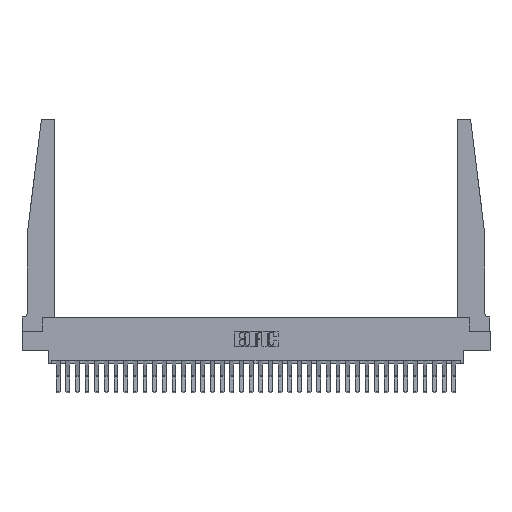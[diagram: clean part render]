
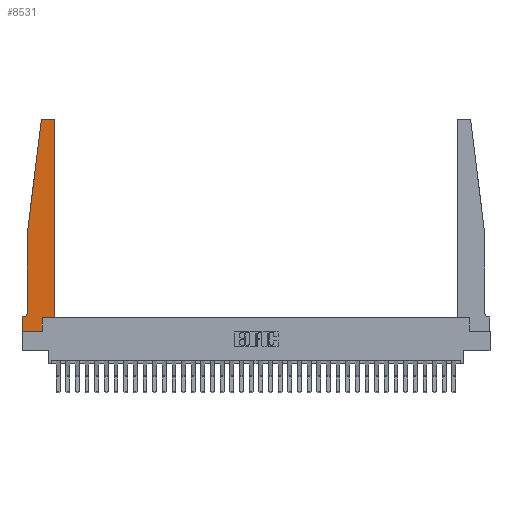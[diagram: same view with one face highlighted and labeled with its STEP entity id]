
A CAD part, top view. The second image highlights one B-rep face of the part: STEP entity #8531.
In plain terms, the highlighted planar face has unit normal (0, 0, 1).
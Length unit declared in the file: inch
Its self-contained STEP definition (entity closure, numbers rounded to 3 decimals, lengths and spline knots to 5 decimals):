
#405 = CARTESIAN_POINT ( 'NONE',  ( 0.27653, 2.75, 0.37 ) ) ;
#960 = EDGE_CURVE ( 'NONE', #11958, #12646, #22011, .T. ) ;
#995 = CARTESIAN_POINT ( 'NONE',  ( 0.065, 0.1875, 0.37 ) ) ;
#1097 = DIRECTION ( 'NONE',  ( -1., 0., 0. ) ) ;
#3001 = DIRECTION ( 'NONE',  ( 0., 0., 1. ) ) ;
#3623 = DIRECTION ( 'NONE',  ( -1., 0., 0. ) ) ;
#4612 = FACE_OUTER_BOUND ( 'NONE', #10465, .T. ) ;
#4649 = VERTEX_POINT ( 'NONE', #405 ) ;
#4705 = EDGE_CURVE ( 'NONE', #25851, #6418, #13183, .T. ) ;
#5505 = VERTEX_POINT ( 'NONE', #24241 ) ;
#5605 = AXIS2_PLACEMENT_3D ( 'NONE', #18018, #3001, #20534 ) ;
#5712 = CARTESIAN_POINT ( 'NONE',  ( 0.395, 2.75, 0.37 ) ) ;
#5839 = CARTESIAN_POINT ( 'NONE',  ( 0.425, 0.18, 0.37 ) ) ;
#5965 = EDGE_CURVE ( 'NONE', #6418, #5505, #16911, .T. ) ;
#6360 = VERTEX_POINT ( 'NONE', #10089 ) ;
#6418 = VERTEX_POINT ( 'NONE', #7805 ) ;
#6749 = CARTESIAN_POINT ( 'NONE',  ( 0., 0., 0.37 ) ) ;
#7024 = CARTESIAN_POINT ( 'NONE',  ( 0.015, 0.1875, 0.37 ) ) ;
#7805 = CARTESIAN_POINT ( 'NONE',  ( 0.065, 1.25, 0.37 ) ) ;
#7877 = EDGE_CURVE ( 'NONE', #22859, #4649, #9354, .T. ) ;
#8269 = VECTOR ( 'NONE', #10960, 39.37008 ) ;
#8531 = ADVANCED_FACE ( 'NONE', ( #4612 ), #10996, .T. ) ;
#8584 = CARTESIAN_POINT ( 'NONE',  ( 0., 0., 0.37 ) ) ;
#9070 = CIRCLE ( 'NONE', #5605, 0.03 ) ;
#9201 = LINE ( 'NONE', #15940, #21704 ) ;
#9333 = CARTESIAN_POINT ( 'NONE',  ( 0.2605, 0.18, 0.37 ) ) ;
#9354 = LINE ( 'NONE', #18634, #16010 ) ;
#10089 = CARTESIAN_POINT ( 'NONE',  ( 0., 0., 0.37 ) ) ;
#10138 = AXIS2_PLACEMENT_3D ( 'NONE', #29573, #14570, #32053 ) ;
#10257 = EDGE_CURVE ( 'NONE', #26370, #11958, #9201, .T. ) ;
#10465 = EDGE_LOOP ( 'NONE', ( #27200, #13073, #22240, #32023, #12083, #15633, #16748, #21264, #22041, #24745, #27992, #22976 ) ) ;
#10863 = DIRECTION ( 'NONE',  ( 0., 1., 0. ) ) ;
#10901 = DIRECTION ( 'NONE',  ( 1., 0., 0. ) ) ;
#10960 = DIRECTION ( 'NONE',  ( 0., -1., 0. ) ) ;
#10984 = CARTESIAN_POINT ( 'NONE',  ( 0.065, 1.25, 0.37 ) ) ;
#10996 = PLANE ( 'NONE',  #29577 ) ;
#11637 = VERTEX_POINT ( 'NONE', #7024 ) ;
#11958 = VERTEX_POINT ( 'NONE', #23150 ) ;
#12083 = ORIENTED_EDGE ( 'NONE', *, *, #22523, .T. ) ;
#12473 = LINE ( 'NONE', #31334, #32404 ) ;
#12572 = EDGE_CURVE ( 'NONE', #11637, #22506, #30091, .T. ) ;
#12646 = VERTEX_POINT ( 'NONE', #21392 ) ;
#13073 = ORIENTED_EDGE ( 'NONE', *, *, #25153, .T. ) ;
#13183 = LINE ( 'NONE', #18083, #25710 ) ;
#13517 = DIRECTION ( 'NONE',  ( 1., 0., 0. ) ) ;
#13553 = CIRCLE ( 'NONE', #10138, 0.05 ) ;
#13858 = LINE ( 'NONE', #6749, #19717 ) ;
#14010 = EDGE_CURVE ( 'NONE', #12646, #22859, #29997, .T. ) ;
#14570 = DIRECTION ( 'NONE',  ( 0., 0., -1. ) ) ;
#14710 = CARTESIAN_POINT ( 'NONE',  ( 0.395, 2.72, 0.37 ) ) ;
#15366 = VECTOR ( 'NONE', #10863, 39.37008 ) ;
#15633 = ORIENTED_EDGE ( 'NONE', *, *, #12572, .T. ) ;
#15940 = CARTESIAN_POINT ( 'NONE',  ( 0.425, 0.18, 0.37 ) ) ;
#16010 = VECTOR ( 'NONE', #3623, 39.37008 ) ;
#16251 = AXIS2_PLACEMENT_3D ( 'NONE', #14710, #32183, #17236 ) ;
#16582 = CARTESIAN_POINT ( 'NONE',  ( 0.2605, 0., 0.37 ) ) ;
#16748 = ORIENTED_EDGE ( 'NONE', *, *, #18124, .T. ) ;
#16911 = LINE ( 'NONE', #10984, #22748 ) ;
#17236 = DIRECTION ( 'NONE',  ( 1., 0., 0. ) ) ;
#18018 = CARTESIAN_POINT ( 'NONE',  ( 0.27653, 2.72, 0.37 ) ) ;
#18083 = CARTESIAN_POINT ( 'NONE',  ( 0.065, 1.25, 0.37 ) ) ;
#18124 = EDGE_CURVE ( 'NONE', #22506, #6360, #28219, .T. ) ;
#18531 = DIRECTION ( 'NONE',  ( 0., -1., 0. ) ) ;
#18634 = CARTESIAN_POINT ( 'NONE',  ( 0.25, 2.75, 0.37 ) ) ;
#18857 = DIRECTION ( 'NONE',  ( 0., 1., 0. ) ) ;
#19717 = VECTOR ( 'NONE', #29288, 39.37008 ) ;
#20215 = EDGE_CURVE ( 'NONE', #27614, #26370, #12473, .T. ) ;
#20534 = DIRECTION ( 'NONE',  ( 1., 0., 0. ) ) ;
#21264 = ORIENTED_EDGE ( 'NONE', *, *, #30290, .T. ) ;
#21392 = CARTESIAN_POINT ( 'NONE',  ( 0.425, 2.72, 0.37 ) ) ;
#21704 = VECTOR ( 'NONE', #10901, 39.37008 ) ;
#22011 = LINE ( 'NONE', #5839, #15366 ) ;
#22041 = ORIENTED_EDGE ( 'NONE', *, *, #20215, .T. ) ;
#22240 = ORIENTED_EDGE ( 'NONE', *, *, #4705, .T. ) ;
#22506 = VERTEX_POINT ( 'NONE', #24411 ) ;
#22523 = EDGE_CURVE ( 'NONE', #5505, #11637, #13553, .T. ) ;
#22748 = VECTOR ( 'NONE', #18531, 39.37008 ) ;
#22859 = VERTEX_POINT ( 'NONE', #5712 ) ;
#22976 = ORIENTED_EDGE ( 'NONE', *, *, #14010, .T. ) ;
#23150 = CARTESIAN_POINT ( 'NONE',  ( 0.425, 0.18, 0.37 ) ) ;
#23424 = VECTOR ( 'NONE', #1097, 39.37008 ) ;
#24241 = CARTESIAN_POINT ( 'NONE',  ( 0.065, 0.2375, 0.37 ) ) ;
#24411 = CARTESIAN_POINT ( 'NONE',  ( 0., 0.1875, 0.37 ) ) ;
#24745 = ORIENTED_EDGE ( 'NONE', *, *, #10257, .T. ) ;
#25153 = EDGE_CURVE ( 'NONE', #4649, #25851, #9070, .T. ) ;
#25636 = DIRECTION ( 'NONE',  ( -0.122, -0.992, 0. ) ) ;
#25710 = VECTOR ( 'NONE', #25636, 39.37008 ) ;
#25851 = VERTEX_POINT ( 'NONE', #25860 ) ;
#25860 = CARTESIAN_POINT ( 'NONE',  ( 0.24675, 2.72367, 0.37 ) ) ;
#26370 = VERTEX_POINT ( 'NONE', #9333 ) ;
#27200 = ORIENTED_EDGE ( 'NONE', *, *, #7877, .T. ) ;
#27614 = VERTEX_POINT ( 'NONE', #16582 ) ;
#27992 = ORIENTED_EDGE ( 'NONE', *, *, #960, .T. ) ;
#28219 = LINE ( 'NONE', #8584, #8269 ) ;
#28406 = CARTESIAN_POINT ( 'NONE',  ( 0., 0.1875, 0.37 ) ) ;
#28522 = DIRECTION ( 'NONE',  ( 0., 0., 1. ) ) ;
#29288 = DIRECTION ( 'NONE',  ( 1., 0., 0. ) ) ;
#29573 = CARTESIAN_POINT ( 'NONE',  ( 0.015, 0.2375, 0.37 ) ) ;
#29577 = AXIS2_PLACEMENT_3D ( 'NONE', #28406, #28522, #13517 ) ;
#29997 = CIRCLE ( 'NONE', #16251, 0.03 ) ;
#30091 = LINE ( 'NONE', #995, #23424 ) ;
#30290 = EDGE_CURVE ( 'NONE', #6360, #27614, #13858, .T. ) ;
#31334 = CARTESIAN_POINT ( 'NONE',  ( 0.2605, 0.18, 0.37 ) ) ;
#32023 = ORIENTED_EDGE ( 'NONE', *, *, #5965, .T. ) ;
#32053 = DIRECTION ( 'NONE',  ( -1., 0., 0. ) ) ;
#32183 = DIRECTION ( 'NONE',  ( 0., 0., 1. ) ) ;
#32404 = VECTOR ( 'NONE', #18857, 39.37008 ) ;
